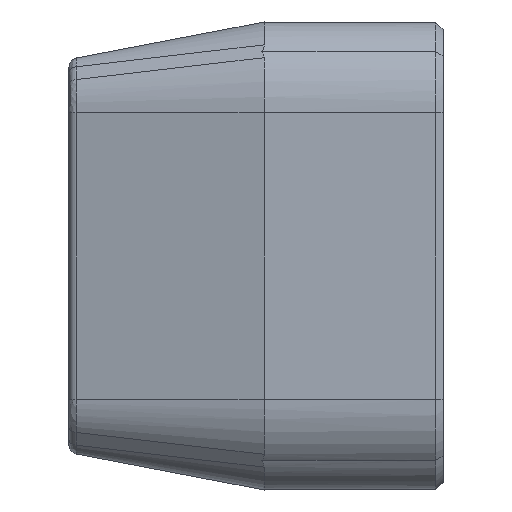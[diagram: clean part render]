
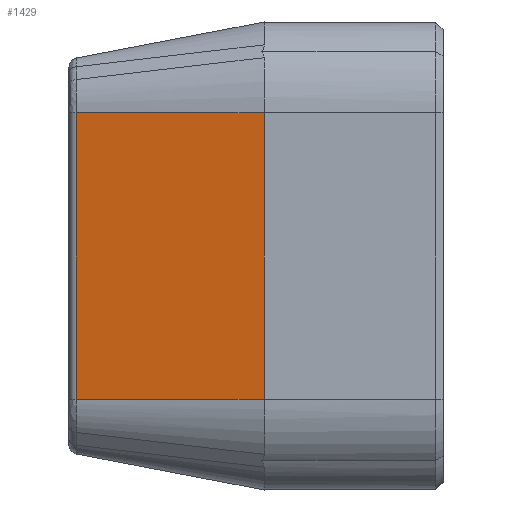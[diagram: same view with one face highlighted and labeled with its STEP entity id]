
A CAD part, front view. The second image highlights one B-rep face of the part: STEP entity #1429.
In plain terms, the highlighted planar face has unit normal (-0.188, -0.982, 0).
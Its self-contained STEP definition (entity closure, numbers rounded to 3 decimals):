
#90 = DIRECTION ( 'NONE',  ( 0., 0., 1. ) ) ;
#130 = ORIENTED_EDGE ( 'NONE', *, *, #5374, .F. ) ;
#350 = VECTOR ( 'NONE', #90, 1000. ) ;
#690 = EDGE_CURVE ( 'NONE', #4273, #3336, #5568, .T. ) ;
#723 = VECTOR ( 'NONE', #6831, 1000. ) ;
#800 = DIRECTION ( 'NONE',  ( -0.188, -0.982, 0. ) ) ;
#825 = CARTESIAN_POINT ( 'NONE',  ( -483., -72.889, -4.183 ) ) ;
#1317 = EDGE_CURVE ( 'NONE', #3515, #3027, #2242, .T. ) ;
#1340 = DIRECTION ( 'NONE',  ( 0.982, -0.188, 0. ) ) ;
#1429 = ADVANCED_FACE ( 'NONE', ( #7307 ), #4526, .T. ) ;
#1582 = CARTESIAN_POINT ( 'NONE',  ( -472.979, -74.811, -8.09 ) ) ;
#1835 = CARTESIAN_POINT ( 'NONE',  ( -483.406, -72.811, 7.372 ) ) ;
#2096 = LINE ( 'NONE', #825, #350 ) ;
#2242 = LINE ( 'NONE', #4334, #7199 ) ;
#2323 = EDGE_CURVE ( 'NONE', #3027, #3336, #3987, .T. ) ;
#2959 = EDGE_LOOP ( 'NONE', ( #130, #7629, #4830, #8105 ) ) ;
#3027 = VERTEX_POINT ( 'NONE', #3936 ) ;
#3336 = VERTEX_POINT ( 'NONE', #6956 ) ;
#3515 = VERTEX_POINT ( 'NONE', #3597 ) ;
#3597 = CARTESIAN_POINT ( 'NONE',  ( -483., -72.889, -7.926 ) ) ;
#3936 = CARTESIAN_POINT ( 'NONE',  ( -472.979, -74.811, -7.926 ) ) ;
#3987 = LINE ( 'NONE', #1582, #723 ) ;
#4046 = VECTOR ( 'NONE', #1340, 1000. ) ;
#4273 = VERTEX_POINT ( 'NONE', #4744 ) ;
#4334 = CARTESIAN_POINT ( 'NONE',  ( -483.406, -72.811, -7.926 ) ) ;
#4387 = AXIS2_PLACEMENT_3D ( 'NONE', #4463, #800, #9690 ) ;
#4463 = CARTESIAN_POINT ( 'NONE',  ( -478.192, -73.811, -8.09 ) ) ;
#4526 = PLANE ( 'NONE',  #4387 ) ;
#4744 = CARTESIAN_POINT ( 'NONE',  ( -483., -72.889, 7.372 ) ) ;
#4830 = ORIENTED_EDGE ( 'NONE', *, *, #2323, .T. ) ;
#5164 = DIRECTION ( 'NONE',  ( 0.982, -0.188, 0. ) ) ;
#5374 = EDGE_CURVE ( 'NONE', #3515, #4273, #2096, .T. ) ;
#5568 = LINE ( 'NONE', #1835, #4046 ) ;
#6831 = DIRECTION ( 'NONE',  ( 0., 0., 1. ) ) ;
#6956 = CARTESIAN_POINT ( 'NONE',  ( -472.979, -74.811, 7.372 ) ) ;
#7199 = VECTOR ( 'NONE', #5164, 1000. ) ;
#7307 = FACE_OUTER_BOUND ( 'NONE', #2959, .T. ) ;
#7629 = ORIENTED_EDGE ( 'NONE', *, *, #1317, .T. ) ;
#8105 = ORIENTED_EDGE ( 'NONE', *, *, #690, .F. ) ;
#9690 = DIRECTION ( 'NONE',  ( 0., 0., 1. ) ) ;
